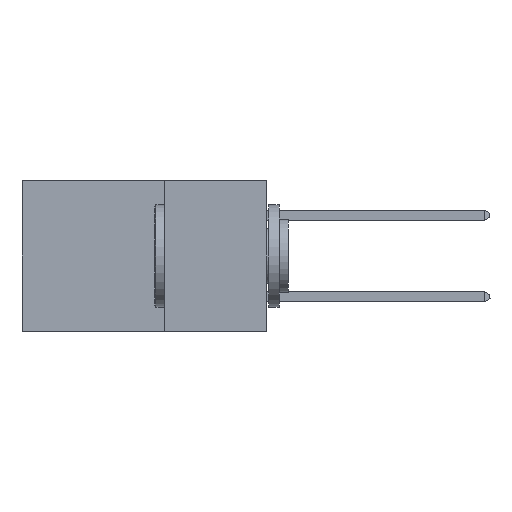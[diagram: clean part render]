
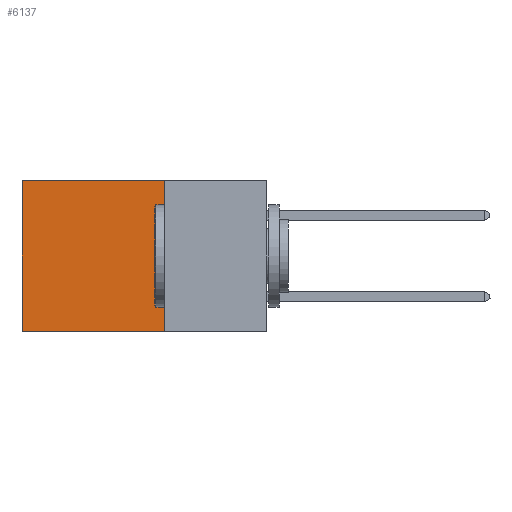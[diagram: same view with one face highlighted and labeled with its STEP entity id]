
A CAD part, left-side view. The second image highlights one B-rep face of the part: STEP entity #6137.
In plain terms, the highlighted planar face has unit normal (-1, 0, 0).
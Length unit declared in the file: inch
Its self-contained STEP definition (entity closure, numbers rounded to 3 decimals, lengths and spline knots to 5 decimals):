
#2479 = LINE ( 'NONE', #8633, #23207 ) ;
#2605 = EDGE_CURVE ( 'NONE', #16488, #6461, #15860, .T. ) ;
#3071 = EDGE_CURVE ( 'NONE', #5894, #6461, #23470, .T. ) ;
#3262 = CARTESIAN_POINT ( 'NONE',  ( 0.2875, 0.6, 0. ) ) ;
#3547 = CARTESIAN_POINT ( 'NONE',  ( 0.2875, 0.6, 0. ) ) ;
#4548 = ORIENTED_EDGE ( 'NONE', *, *, #2605, .T. ) ;
#5365 = CARTESIAN_POINT ( 'NONE',  ( 0.2875, 0.25, -0.37 ) ) ;
#5894 = VERTEX_POINT ( 'NONE', #17785 ) ;
#6137 = ADVANCED_FACE ( 'NONE', ( #8457 ), #19463, .F. ) ;
#6238 = CARTESIAN_POINT ( 'NONE',  ( 0.2875, 0.25, 0. ) ) ;
#6461 = VERTEX_POINT ( 'NONE', #22223 ) ;
#7666 = DIRECTION ( 'NONE',  ( 0., 1., 0. ) ) ;
#7987 = EDGE_CURVE ( 'NONE', #27468, #5894, #2479, .T. ) ;
#8457 = FACE_OUTER_BOUND ( 'NONE', #9622, .T. ) ;
#8633 = CARTESIAN_POINT ( 'NONE',  ( 0.2875, 0.25, 0. ) ) ;
#9622 = EDGE_LOOP ( 'NONE', ( #4548, #16776, #25295, #11206 ) ) ;
#10018 = CARTESIAN_POINT ( 'NONE',  ( 0.2875, 0.25, 0. ) ) ;
#10670 = DIRECTION ( 'NONE',  ( 0., 0., -1. ) ) ;
#11206 = ORIENTED_EDGE ( 'NONE', *, *, #23957, .T. ) ;
#12514 = DIRECTION ( 'NONE',  ( 0., 0., -1. ) ) ;
#14830 = DIRECTION ( 'NONE',  ( 1., 0., 0. ) ) ;
#15860 = LINE ( 'NONE', #3547, #20344 ) ;
#16488 = VERTEX_POINT ( 'NONE', #3262 ) ;
#16776 = ORIENTED_EDGE ( 'NONE', *, *, #3071, .F. ) ;
#17437 = DIRECTION ( 'NONE',  ( 0., 0., -1. ) ) ;
#17602 = VECTOR ( 'NONE', #7666, 39.37008 ) ;
#17785 = CARTESIAN_POINT ( 'NONE',  ( 0.2875, 0.25, -0.37 ) ) ;
#17911 = LINE ( 'NONE', #10018, #23090 ) ;
#19463 = PLANE ( 'NONE',  #28294 ) ;
#20344 = VECTOR ( 'NONE', #12514, 39.37008 ) ;
#22223 = CARTESIAN_POINT ( 'NONE',  ( 0.2875, 0.6, -0.37 ) ) ;
#23090 = VECTOR ( 'NONE', #27535, 39.37008 ) ;
#23207 = VECTOR ( 'NONE', #17437, 39.37008 ) ;
#23470 = LINE ( 'NONE', #5365, #17602 ) ;
#23957 = EDGE_CURVE ( 'NONE', #27468, #16488, #17911, .T. ) ;
#25295 = ORIENTED_EDGE ( 'NONE', *, *, #7987, .F. ) ;
#26467 = CARTESIAN_POINT ( 'NONE',  ( 0.2875, 0.25, 0. ) ) ;
#27468 = VERTEX_POINT ( 'NONE', #26467 ) ;
#27535 = DIRECTION ( 'NONE',  ( 0., 1., 0. ) ) ;
#28294 = AXIS2_PLACEMENT_3D ( 'NONE', #6238, #14830, #10670 ) ;
